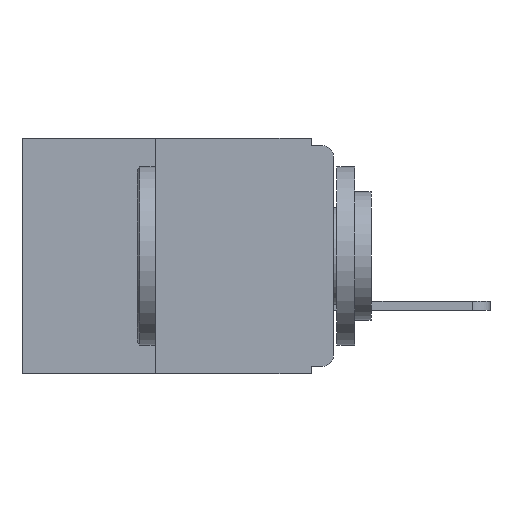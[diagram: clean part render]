
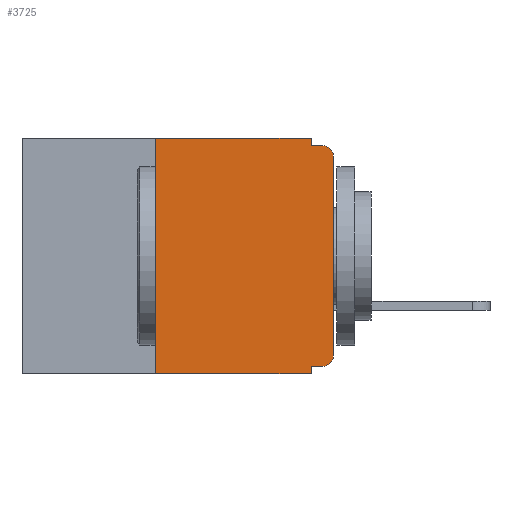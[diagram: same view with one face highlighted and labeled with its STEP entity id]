
A CAD part, left-side view. The second image highlights one B-rep face of the part: STEP entity #3725.
In plain terms, the highlighted planar face has unit normal (-1, 0, 0).
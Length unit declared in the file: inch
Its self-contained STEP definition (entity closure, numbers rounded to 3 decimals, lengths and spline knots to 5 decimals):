
#121 = VECTOR ( 'NONE', #6006, 39.37008 ) ;
#149 = LINE ( 'NONE', #7074, #8890 ) ;
#789 = CARTESIAN_POINT ( 'NONE',  ( 0., 0., -0.025 ) ) ;
#1006 = EDGE_CURVE ( 'NONE', #6807, #19132, #3818, .T. ) ;
#1325 = CARTESIAN_POINT ( 'NONE',  ( 0., 0.031, -0.32 ) ) ;
#1434 = DIRECTION ( 'NONE',  ( -1., 0., 0. ) ) ;
#1542 = CARTESIAN_POINT ( 'NONE',  ( 0., 0.015, -0.305 ) ) ;
#1874 = EDGE_CURVE ( 'NONE', #20167, #21282, #11083, .T. ) ;
#1986 = PLANE ( 'NONE',  #15044 ) ;
#2187 = CARTESIAN_POINT ( 'NONE',  ( 0., 0.015, -0.32 ) ) ;
#2346 = ORIENTED_EDGE ( 'NONE', *, *, #17796, .T. ) ;
#2448 = CARTESIAN_POINT ( 'NONE',  ( 0., 0.031, -0.01 ) ) ;
#2900 = CARTESIAN_POINT ( 'NONE',  ( 0., 0., -0.305 ) ) ;
#3226 = VECTOR ( 'NONE', #17261, 39.37008 ) ;
#3725 = ADVANCED_FACE ( 'NONE', ( #4000 ), #1986, .F. ) ;
#3818 = CIRCLE ( 'NONE', #9690, 0.015 ) ;
#3927 = VERTEX_POINT ( 'NONE', #2448 ) ;
#4000 = FACE_OUTER_BOUND ( 'NONE', #4596, .T. ) ;
#4224 = CARTESIAN_POINT ( 'NONE',  ( 0., 0.015, -0.01 ) ) ;
#4372 = CARTESIAN_POINT ( 'NONE',  ( 0., 0.031, -0.33 ) ) ;
#4460 = CARTESIAN_POINT ( 'NONE',  ( 0., 0., 0. ) ) ;
#4596 = EDGE_LOOP ( 'NONE', ( #2346, #17455, #10521, #15883, #12639, #21062, #18943, #15169, #9353, #17362 ) ) ;
#5068 = CARTESIAN_POINT ( 'NONE',  ( 0., 0.015, -0.025 ) ) ;
#5278 = EDGE_CURVE ( 'NONE', #16487, #20167, #15737, .T. ) ;
#5493 = DIRECTION ( 'NONE',  ( 0., 0., -1. ) ) ;
#5916 = VECTOR ( 'NONE', #18225, 39.37008 ) ;
#6006 = DIRECTION ( 'NONE',  ( 0., -1., 0. ) ) ;
#6229 = CARTESIAN_POINT ( 'NONE',  ( 0., 0.437, 0. ) ) ;
#6573 = DIRECTION ( 'NONE',  ( 0., 0., 1. ) ) ;
#6627 = CIRCLE ( 'NONE', #14314, 0.015 ) ;
#6807 = VERTEX_POINT ( 'NONE', #2187 ) ;
#6819 = DIRECTION ( 'NONE',  ( 0., 0., -1. ) ) ;
#7039 = VECTOR ( 'NONE', #10640, 39.37008 ) ;
#7074 = CARTESIAN_POINT ( 'NONE',  ( 0., 0.031, 0. ) ) ;
#7590 = LINE ( 'NONE', #8924, #7039 ) ;
#7971 = DIRECTION ( 'NONE',  ( 0., -1., 0. ) ) ;
#8819 = DIRECTION ( 'NONE',  ( 0., 0., -1. ) ) ;
#8890 = VECTOR ( 'NONE', #8819, 39.37008 ) ;
#8924 = CARTESIAN_POINT ( 'NONE',  ( 0., 0., -0.32 ) ) ;
#9353 = ORIENTED_EDGE ( 'NONE', *, *, #20595, .F. ) ;
#9690 = AXIS2_PLACEMENT_3D ( 'NONE', #1542, #1434, #12989 ) ;
#10521 = ORIENTED_EDGE ( 'NONE', *, *, #17081, .F. ) ;
#10640 = DIRECTION ( 'NONE',  ( 0., 1., 0. ) ) ;
#10657 = VECTOR ( 'NONE', #6573, 39.37008 ) ;
#10848 = CARTESIAN_POINT ( 'NONE',  ( 0., 0.031, -0.33 ) ) ;
#11031 = LINE ( 'NONE', #4460, #5916 ) ;
#11083 = LINE ( 'NONE', #6229, #19121 ) ;
#11246 = VERTEX_POINT ( 'NONE', #1325 ) ;
#11605 = CARTESIAN_POINT ( 'NONE',  ( 0., 0.25, -0.33 ) ) ;
#11654 = VERTEX_POINT ( 'NONE', #4224 ) ;
#11678 = VERTEX_POINT ( 'NONE', #4372 ) ;
#12107 = EDGE_CURVE ( 'NONE', #11246, #11678, #21477, .T. ) ;
#12489 = EDGE_CURVE ( 'NONE', #21282, #3927, #149, .T. ) ;
#12550 = DIRECTION ( 'NONE',  ( 0., 0., -1. ) ) ;
#12639 = ORIENTED_EDGE ( 'NONE', *, *, #1874, .F. ) ;
#12989 = DIRECTION ( 'NONE',  ( 0., 0., -1. ) ) ;
#13953 = LINE ( 'NONE', #16276, #121 ) ;
#14058 = CARTESIAN_POINT ( 'NONE',  ( 0., 0.437, 0. ) ) ;
#14314 = AXIS2_PLACEMENT_3D ( 'NONE', #5068, #17093, #6819 ) ;
#14440 = CARTESIAN_POINT ( 'NONE',  ( 0., 0.031, 0. ) ) ;
#15044 = AXIS2_PLACEMENT_3D ( 'NONE', #14058, #15773, #5493 ) ;
#15064 = EDGE_CURVE ( 'NONE', #21996, #11654, #6627, .T. ) ;
#15169 = ORIENTED_EDGE ( 'NONE', *, *, #12107, .F. ) ;
#15737 = LINE ( 'NONE', #11605, #10657 ) ;
#15773 = DIRECTION ( 'NONE',  ( 1., 0., 0. ) ) ;
#15833 = CARTESIAN_POINT ( 'NONE',  ( 0., 0.25, -0.33 ) ) ;
#15883 = ORIENTED_EDGE ( 'NONE', *, *, #12489, .F. ) ;
#16276 = CARTESIAN_POINT ( 'NONE',  ( 0., 0.437, -0.33 ) ) ;
#16321 = CARTESIAN_POINT ( 'NONE',  ( 0., 0.25, 0. ) ) ;
#16487 = VERTEX_POINT ( 'NONE', #15833 ) ;
#16963 = VECTOR ( 'NONE', #12550, 39.37008 ) ;
#17081 = EDGE_CURVE ( 'NONE', #3927, #11654, #20967, .T. ) ;
#17093 = DIRECTION ( 'NONE',  ( -1., 0., 0. ) ) ;
#17261 = DIRECTION ( 'NONE',  ( 0., -1., 0. ) ) ;
#17362 = ORIENTED_EDGE ( 'NONE', *, *, #1006, .T. ) ;
#17455 = ORIENTED_EDGE ( 'NONE', *, *, #15064, .T. ) ;
#17796 = EDGE_CURVE ( 'NONE', #19132, #21996, #11031, .T. ) ;
#18225 = DIRECTION ( 'NONE',  ( 0., 0., 1. ) ) ;
#18943 = ORIENTED_EDGE ( 'NONE', *, *, #21964, .T. ) ;
#19050 = CARTESIAN_POINT ( 'NONE',  ( 0., 0., -0.01 ) ) ;
#19121 = VECTOR ( 'NONE', #7971, 39.37008 ) ;
#19132 = VERTEX_POINT ( 'NONE', #2900 ) ;
#20167 = VERTEX_POINT ( 'NONE', #16321 ) ;
#20595 = EDGE_CURVE ( 'NONE', #6807, #11246, #7590, .T. ) ;
#20967 = LINE ( 'NONE', #19050, #3226 ) ;
#21062 = ORIENTED_EDGE ( 'NONE', *, *, #5278, .F. ) ;
#21282 = VERTEX_POINT ( 'NONE', #14440 ) ;
#21477 = LINE ( 'NONE', #10848, #16963 ) ;
#21964 = EDGE_CURVE ( 'NONE', #16487, #11678, #13953, .T. ) ;
#21996 = VERTEX_POINT ( 'NONE', #789 ) ;
